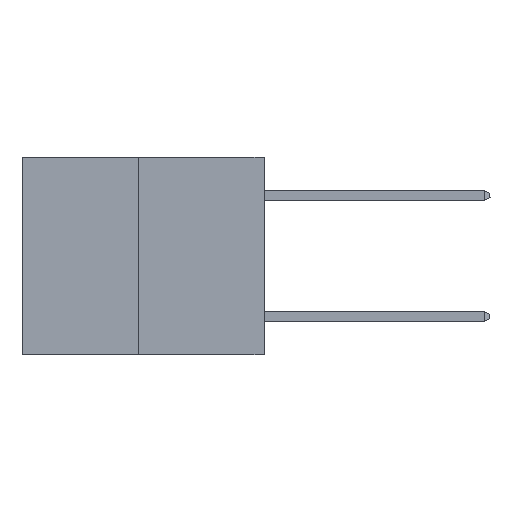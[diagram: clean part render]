
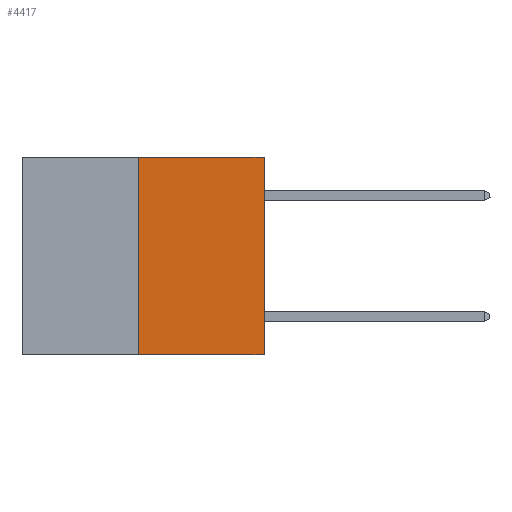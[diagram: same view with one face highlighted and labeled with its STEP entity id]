
A CAD part, left-side view. The second image highlights one B-rep face of the part: STEP entity #4417.
In plain terms, the highlighted planar face has unit normal (-1, 0, 0).
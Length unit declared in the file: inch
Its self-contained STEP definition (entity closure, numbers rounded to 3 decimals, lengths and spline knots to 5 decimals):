
#54 = DIRECTION ( 'NONE',  ( 0., 0., 1. ) ) ;
#1661 = VERTEX_POINT ( 'NONE', #3844 ) ;
#1920 = ORIENTED_EDGE ( 'NONE', *, *, #13196, .F. ) ;
#2369 = DIRECTION ( 'NONE',  ( 0., -1., 0. ) ) ;
#3209 = VECTOR ( 'NONE', #2369, 39.37008 ) ;
#3313 = CARTESIAN_POINT ( 'NONE',  ( 0., 0.312, -0.49 ) ) ;
#3795 = VERTEX_POINT ( 'NONE', #12615 ) ;
#3844 = CARTESIAN_POINT ( 'NONE',  ( 0., 0., 0. ) ) ;
#4417 = ADVANCED_FACE ( 'NONE', ( #19308 ), #19500, .F. ) ;
#5256 = LINE ( 'NONE', #26782, #15494 ) ;
#8243 = DIRECTION ( 'NONE',  ( 1., 0., 0. ) ) ;
#8612 = AXIS2_PLACEMENT_3D ( 'NONE', #21339, #8243, #10677 ) ;
#8825 = VECTOR ( 'NONE', #17621, 39.37008 ) ;
#9320 = LINE ( 'NONE', #27927, #22299 ) ;
#9518 = ORIENTED_EDGE ( 'NONE', *, *, #11590, .F. ) ;
#9751 = EDGE_CURVE ( 'NONE', #27043, #1661, #10824, .T. ) ;
#10677 = DIRECTION ( 'NONE',  ( 0., 0., -1. ) ) ;
#10824 = LINE ( 'NONE', #22228, #8825 ) ;
#11590 = EDGE_CURVE ( 'NONE', #3795, #1661, #14845, .T. ) ;
#12615 = CARTESIAN_POINT ( 'NONE',  ( 0., 0.312, 0. ) ) ;
#13196 = EDGE_CURVE ( 'NONE', #19545, #3795, #9320, .T. ) ;
#14845 = LINE ( 'NONE', #15015, #3209 ) ;
#15015 = CARTESIAN_POINT ( 'NONE',  ( 0., 0.6, 0. ) ) ;
#15494 = VECTOR ( 'NONE', #16119, 39.37008 ) ;
#16119 = DIRECTION ( 'NONE',  ( 0., -1., 0. ) ) ;
#17621 = DIRECTION ( 'NONE',  ( 0., 0., 1. ) ) ;
#19308 = FACE_OUTER_BOUND ( 'NONE', #19489, .T. ) ;
#19489 = EDGE_LOOP ( 'NONE', ( #1920, #28091, #19605, #9518 ) ) ;
#19500 = PLANE ( 'NONE',  #8612 ) ;
#19545 = VERTEX_POINT ( 'NONE', #3313 ) ;
#19605 = ORIENTED_EDGE ( 'NONE', *, *, #9751, .T. ) ;
#21339 = CARTESIAN_POINT ( 'NONE',  ( 0., 0.6, 0. ) ) ;
#22228 = CARTESIAN_POINT ( 'NONE',  ( 0., 0., 0. ) ) ;
#22299 = VECTOR ( 'NONE', #54, 39.37008 ) ;
#22760 = EDGE_CURVE ( 'NONE', #19545, #27043, #5256, .T. ) ;
#26782 = CARTESIAN_POINT ( 'NONE',  ( 0., 0.6, -0.49 ) ) ;
#27043 = VERTEX_POINT ( 'NONE', #27621 ) ;
#27621 = CARTESIAN_POINT ( 'NONE',  ( 0., 0., -0.49 ) ) ;
#27927 = CARTESIAN_POINT ( 'NONE',  ( 0., 0.312, -0.49 ) ) ;
#28091 = ORIENTED_EDGE ( 'NONE', *, *, #22760, .T. ) ;
